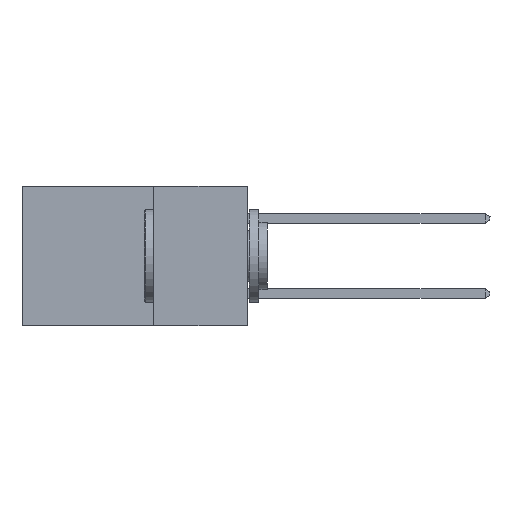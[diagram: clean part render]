
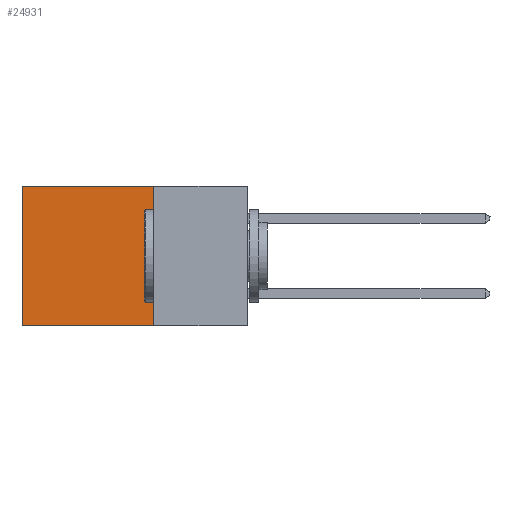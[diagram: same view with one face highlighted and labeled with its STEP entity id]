
A CAD part, left-side view. The second image highlights one B-rep face of the part: STEP entity #24931.
In plain terms, the highlighted planar face has unit normal (-1, 0, 0).
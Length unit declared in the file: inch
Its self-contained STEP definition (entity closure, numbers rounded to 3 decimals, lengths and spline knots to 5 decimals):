
#235 = LINE ( 'NONE', #17688, #23037 ) ;
#428 = LINE ( 'NONE', #2251, #6527 ) ;
#2251 = CARTESIAN_POINT ( 'NONE',  ( 0.2615, 0.25, 0. ) ) ;
#2814 = VERTEX_POINT ( 'NONE', #14300 ) ;
#4194 = VECTOR ( 'NONE', #15880, 39.37008 ) ;
#4489 = VERTEX_POINT ( 'NONE', #12268 ) ;
#5296 = VERTEX_POINT ( 'NONE', #22053 ) ;
#6395 = DIRECTION ( 'NONE',  ( 0., 0., -1. ) ) ;
#6527 = VECTOR ( 'NONE', #23609, 39.37008 ) ;
#7294 = VERTEX_POINT ( 'NONE', #21721 ) ;
#7768 = EDGE_CURVE ( 'NONE', #5296, #4489, #428, .T. ) ;
#8975 = ORIENTED_EDGE ( 'NONE', *, *, #23690, .F. ) ;
#12268 = CARTESIAN_POINT ( 'NONE',  ( 0.2615, 0.6, 0. ) ) ;
#13804 = ORIENTED_EDGE ( 'NONE', *, *, #14585, .T. ) ;
#14038 = FACE_OUTER_BOUND ( 'NONE', #23004, .T. ) ;
#14300 = CARTESIAN_POINT ( 'NONE',  ( 0.2615, 0.6, -0.37 ) ) ;
#14585 = EDGE_CURVE ( 'NONE', #4489, #2814, #22584, .T. ) ;
#14936 = EDGE_CURVE ( 'NONE', #7294, #2814, #235, .T. ) ;
#14939 = AXIS2_PLACEMENT_3D ( 'NONE', #20629, #20501, #16427 ) ;
#15288 = DIRECTION ( 'NONE',  ( 0., 1., 0. ) ) ;
#15880 = DIRECTION ( 'NONE',  ( 0., 0., -1. ) ) ;
#16427 = DIRECTION ( 'NONE',  ( 0., 0., -1. ) ) ;
#17688 = CARTESIAN_POINT ( 'NONE',  ( 0.2615, 0.25, -0.37 ) ) ;
#19246 = ORIENTED_EDGE ( 'NONE', *, *, #14936, .F. ) ;
#20501 = DIRECTION ( 'NONE',  ( 1., 0., 0. ) ) ;
#20629 = CARTESIAN_POINT ( 'NONE',  ( 0.2615, 0.25, -0.37 ) ) ;
#21721 = CARTESIAN_POINT ( 'NONE',  ( 0.2615, 0.25, -0.37 ) ) ;
#22053 = CARTESIAN_POINT ( 'NONE',  ( 0.2615, 0.25, 0. ) ) ;
#22584 = LINE ( 'NONE', #26930, #4194 ) ;
#23004 = EDGE_LOOP ( 'NONE', ( #13804, #19246, #8975, #24710 ) ) ;
#23037 = VECTOR ( 'NONE', #15288, 39.37008 ) ;
#23609 = DIRECTION ( 'NONE',  ( 0., 1., 0. ) ) ;
#23690 = EDGE_CURVE ( 'NONE', #5296, #7294, #27617, .T. ) ;
#24410 = PLANE ( 'NONE',  #14939 ) ;
#24710 = ORIENTED_EDGE ( 'NONE', *, *, #7768, .T. ) ;
#24931 = ADVANCED_FACE ( 'NONE', ( #14038 ), #24410, .F. ) ;
#26930 = CARTESIAN_POINT ( 'NONE',  ( 0.2615, 0.6, -0.37 ) ) ;
#27425 = VECTOR ( 'NONE', #6395, 39.37008 ) ;
#27464 = CARTESIAN_POINT ( 'NONE',  ( 0.2615, 0.25, -0.37 ) ) ;
#27617 = LINE ( 'NONE', #27464, #27425 ) ;
